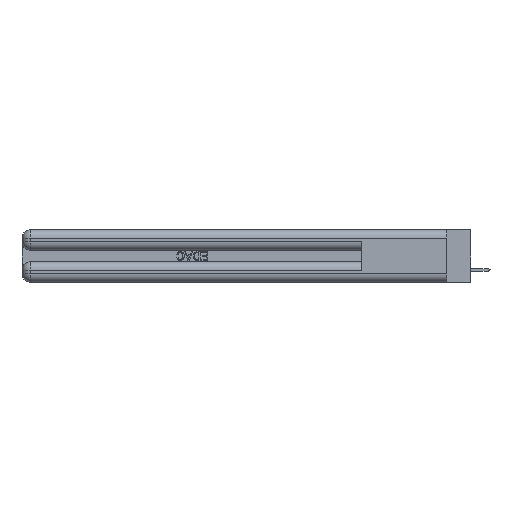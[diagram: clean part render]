
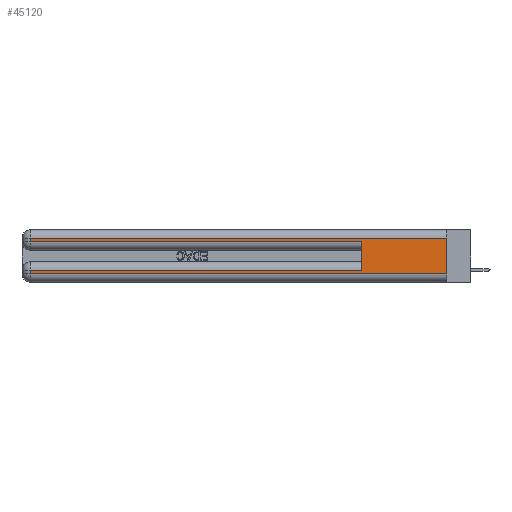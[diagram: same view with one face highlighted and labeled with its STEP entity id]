
A CAD part, left-side view. The second image highlights one B-rep face of the part: STEP entity #45120.
In plain terms, the highlighted planar face has unit normal (-1, 0, 0).
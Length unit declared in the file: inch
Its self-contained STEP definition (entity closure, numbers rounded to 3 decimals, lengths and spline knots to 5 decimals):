
#510 = AXIS2_PLACEMENT_3D ( 'NONE', #3406, #32754, #44033 ) ;
#1059 = DIRECTION ( 'NONE',  ( 0., 0., 1. ) ) ;
#1291 = DIRECTION ( 'NONE',  ( 0., 1., 0. ) ) ;
#2636 = CARTESIAN_POINT ( 'NONE',  ( 0., 2.94, 0.37 ) ) ;
#3406 = CARTESIAN_POINT ( 'NONE',  ( 0., 0., 0.37 ) ) ;
#3678 = VERTEX_POINT ( 'NONE', #35568 ) ;
#4453 = VERTEX_POINT ( 'NONE', #10943 ) ;
#4672 = CARTESIAN_POINT ( 'NONE',  ( 0., 0.6, 0.145 ) ) ;
#5892 = EDGE_CURVE ( 'NONE', #45629, #3678, #36904, .T. ) ;
#7181 = VECTOR ( 'NONE', #16907, 39.37008 ) ;
#7482 = LINE ( 'NONE', #29126, #38967 ) ;
#9000 = LINE ( 'NONE', #37353, #44998 ) ;
#9179 = VERTEX_POINT ( 'NONE', #41948 ) ;
#10330 = ORIENTED_EDGE ( 'NONE', *, *, #5892, .F. ) ;
#10475 = EDGE_CURVE ( 'NONE', #36939, #26591, #12459, .T. ) ;
#10557 = LINE ( 'NONE', #28839, #36632 ) ;
#10943 = CARTESIAN_POINT ( 'NONE',  ( 0., 2.94, 0.06 ) ) ;
#10981 = CARTESIAN_POINT ( 'NONE',  ( 0., 0., 0.06 ) ) ;
#12459 = LINE ( 'NONE', #33864, #22461 ) ;
#13776 = LINE ( 'NONE', #35633, #7181 ) ;
#14163 = VECTOR ( 'NONE', #29114, 39.37008 ) ;
#14188 = EDGE_CURVE ( 'NONE', #15133, #14611, #35820, .T. ) ;
#14611 = VERTEX_POINT ( 'NONE', #15747 ) ;
#15133 = VERTEX_POINT ( 'NONE', #46656 ) ;
#15747 = CARTESIAN_POINT ( 'NONE',  ( 0., 2.94, 0.285 ) ) ;
#16907 = DIRECTION ( 'NONE',  ( 0., 1., 0. ) ) ;
#18602 = ORIENTED_EDGE ( 'NONE', *, *, #10475, .F. ) ;
#18705 = DIRECTION ( 'NONE',  ( 0., -1., 0. ) ) ;
#18757 = DIRECTION ( 'NONE',  ( 0., -1., 0. ) ) ;
#21684 = FACE_OUTER_BOUND ( 'NONE', #30510, .T. ) ;
#22117 = CARTESIAN_POINT ( 'NONE',  ( 0., 2.94, 0.37 ) ) ;
#22461 = VECTOR ( 'NONE', #30027, 39.37008 ) ;
#23355 = EDGE_CURVE ( 'NONE', #4453, #26591, #7482, .T. ) ;
#23750 = EDGE_CURVE ( 'NONE', #14611, #3678, #10557, .T. ) ;
#24083 = LINE ( 'NONE', #2636, #32088 ) ;
#25062 = ORIENTED_EDGE ( 'NONE', *, *, #36725, .T. ) ;
#26591 = VERTEX_POINT ( 'NONE', #10981 ) ;
#26949 = ORIENTED_EDGE ( 'NONE', *, *, #42517, .T. ) ;
#27759 = ORIENTED_EDGE ( 'NONE', *, *, #23750, .T. ) ;
#28839 = CARTESIAN_POINT ( 'NONE',  ( 0., 0., 0.285 ) ) ;
#29114 = DIRECTION ( 'NONE',  ( 0., 0., -1. ) ) ;
#29126 = CARTESIAN_POINT ( 'NONE',  ( 0., 0., 0.06 ) ) ;
#30027 = DIRECTION ( 'NONE',  ( 0., 0., -1. ) ) ;
#30410 = ORIENTED_EDGE ( 'NONE', *, *, #41898, .T. ) ;
#30510 = EDGE_LOOP ( 'NONE', ( #18602, #30410, #39857, #27759, #10330, #25062, #26949, #38168 ) ) ;
#31522 = DIRECTION ( 'NONE',  ( 0., 0., -1. ) ) ;
#32088 = VECTOR ( 'NONE', #31522, 39.37008 ) ;
#32754 = DIRECTION ( 'NONE',  ( 1., 0., 0. ) ) ;
#33864 = CARTESIAN_POINT ( 'NONE',  ( 0., 0., 0.37 ) ) ;
#35568 = CARTESIAN_POINT ( 'NONE',  ( 0., 0.6, 0.285 ) ) ;
#35633 = CARTESIAN_POINT ( 'NONE',  ( 0., 0., 0.085 ) ) ;
#35820 = LINE ( 'NONE', #22117, #14163 ) ;
#36345 = PLANE ( 'NONE',  #510 ) ;
#36632 = VECTOR ( 'NONE', #18705, 39.37008 ) ;
#36725 = EDGE_CURVE ( 'NONE', #45629, #9179, #13776, .T. ) ;
#36904 = LINE ( 'NONE', #4672, #39028 ) ;
#36939 = VERTEX_POINT ( 'NONE', #38502 ) ;
#37353 = CARTESIAN_POINT ( 'NONE',  ( 0., 0., 0.31 ) ) ;
#38168 = ORIENTED_EDGE ( 'NONE', *, *, #23355, .T. ) ;
#38502 = CARTESIAN_POINT ( 'NONE',  ( 0., 0., 0.31 ) ) ;
#38967 = VECTOR ( 'NONE', #18757, 39.37008 ) ;
#39028 = VECTOR ( 'NONE', #1059, 39.37008 ) ;
#39857 = ORIENTED_EDGE ( 'NONE', *, *, #14188, .T. ) ;
#41898 = EDGE_CURVE ( 'NONE', #36939, #15133, #9000, .T. ) ;
#41948 = CARTESIAN_POINT ( 'NONE',  ( 0., 2.94, 0.085 ) ) ;
#42517 = EDGE_CURVE ( 'NONE', #9179, #4453, #24083, .T. ) ;
#44033 = DIRECTION ( 'NONE',  ( 0., 0., -1. ) ) ;
#44998 = VECTOR ( 'NONE', #1291, 39.37008 ) ;
#45120 = ADVANCED_FACE ( 'NONE', ( #21684 ), #36345, .F. ) ;
#45629 = VERTEX_POINT ( 'NONE', #46115 ) ;
#46115 = CARTESIAN_POINT ( 'NONE',  ( 0., 0.6, 0.085 ) ) ;
#46656 = CARTESIAN_POINT ( 'NONE',  ( 0., 2.94, 0.31 ) ) ;
